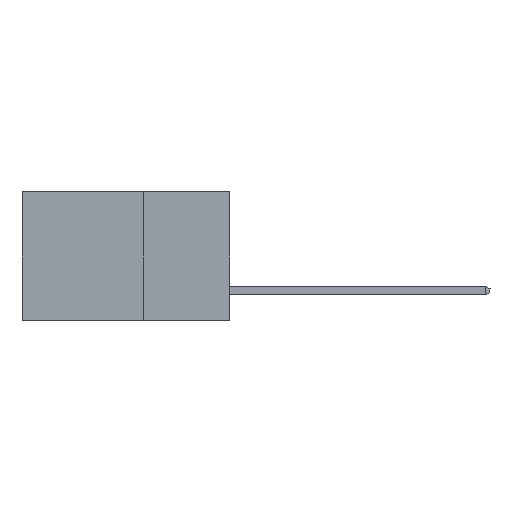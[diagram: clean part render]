
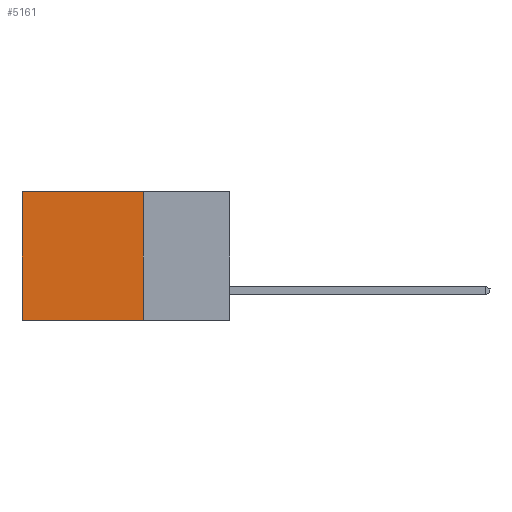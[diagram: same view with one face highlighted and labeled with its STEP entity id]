
A CAD part, left-side view. The second image highlights one B-rep face of the part: STEP entity #5161.
In plain terms, the highlighted planar face has unit normal (-1, 0, 0).
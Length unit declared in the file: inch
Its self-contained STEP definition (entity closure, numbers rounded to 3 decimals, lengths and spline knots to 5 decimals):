
#35 = CARTESIAN_POINT ( 'NONE',  ( 0.2615, 0.6, -0.37 ) ) ;
#76 = EDGE_CURVE ( 'NONE', #6805, #6786, #541, .T. ) ;
#541 = LINE ( 'NONE', #13327, #10309 ) ;
#590 = DIRECTION ( 'NONE',  ( 0., 1., 0. ) ) ;
#1802 = DIRECTION ( 'NONE',  ( 0., 0., -1. ) ) ;
#1931 = ORIENTED_EDGE ( 'NONE', *, *, #11568, .T. ) ;
#2744 = EDGE_CURVE ( 'NONE', #4774, #8734, #6013, .T. ) ;
#3733 = CARTESIAN_POINT ( 'NONE',  ( 0.2615, 0.25, -0.37 ) ) ;
#4348 = FACE_OUTER_BOUND ( 'NONE', #10248, .T. ) ;
#4414 = CARTESIAN_POINT ( 'NONE',  ( 0.2615, 0.25, -0.37 ) ) ;
#4774 = VERTEX_POINT ( 'NONE', #9541 ) ;
#5161 = ADVANCED_FACE ( 'NONE', ( #4348 ), #9517, .F. ) ;
#5464 = CARTESIAN_POINT ( 'NONE',  ( 0.2615, 0.25, -0.37 ) ) ;
#5747 = ORIENTED_EDGE ( 'NONE', *, *, #2744, .T. ) ;
#6013 = LINE ( 'NONE', #8949, #7456 ) ;
#6786 = VERTEX_POINT ( 'NONE', #35 ) ;
#6805 = VERTEX_POINT ( 'NONE', #5464 ) ;
#6902 = ORIENTED_EDGE ( 'NONE', *, *, #8685, .F. ) ;
#7456 = VECTOR ( 'NONE', #590, 39.37008 ) ;
#8002 = LINE ( 'NONE', #8068, #11709 ) ;
#8068 = CARTESIAN_POINT ( 'NONE',  ( 0.2615, 0.6, -0.37 ) ) ;
#8104 = VECTOR ( 'NONE', #13348, 39.37008 ) ;
#8541 = DIRECTION ( 'NONE',  ( 0., 0., -1. ) ) ;
#8685 = EDGE_CURVE ( 'NONE', #4774, #6805, #11243, .T. ) ;
#8734 = VERTEX_POINT ( 'NONE', #13555 ) ;
#8949 = CARTESIAN_POINT ( 'NONE',  ( 0.2615, 0.25, 0. ) ) ;
#9446 = DIRECTION ( 'NONE',  ( 1., 0., 0. ) ) ;
#9517 = PLANE ( 'NONE',  #10980 ) ;
#9541 = CARTESIAN_POINT ( 'NONE',  ( 0.2615, 0.25, 0. ) ) ;
#10248 = EDGE_LOOP ( 'NONE', ( #1931, #12087, #6902, #5747 ) ) ;
#10309 = VECTOR ( 'NONE', #13184, 39.37008 ) ;
#10980 = AXIS2_PLACEMENT_3D ( 'NONE', #4414, #9446, #8541 ) ;
#11243 = LINE ( 'NONE', #3733, #8104 ) ;
#11568 = EDGE_CURVE ( 'NONE', #8734, #6786, #8002, .T. ) ;
#11709 = VECTOR ( 'NONE', #1802, 39.37008 ) ;
#12087 = ORIENTED_EDGE ( 'NONE', *, *, #76, .F. ) ;
#13184 = DIRECTION ( 'NONE',  ( 0., 1., 0. ) ) ;
#13327 = CARTESIAN_POINT ( 'NONE',  ( 0.2615, 0.25, -0.37 ) ) ;
#13348 = DIRECTION ( 'NONE',  ( 0., 0., -1. ) ) ;
#13555 = CARTESIAN_POINT ( 'NONE',  ( 0.2615, 0.6, 0. ) ) ;
